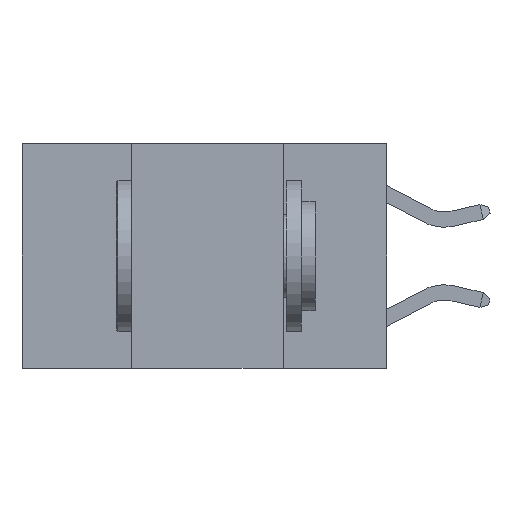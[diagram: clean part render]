
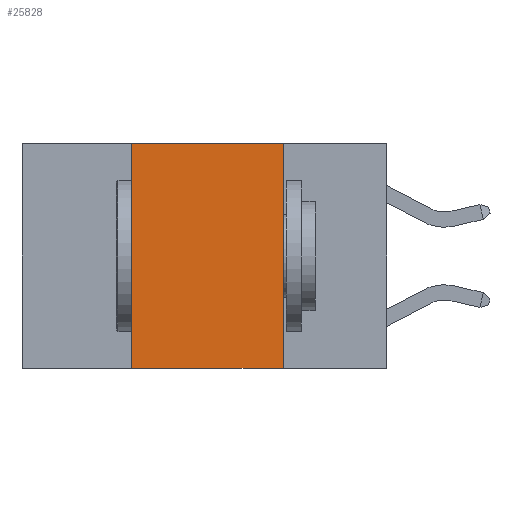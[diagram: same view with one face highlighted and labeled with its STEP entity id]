
A CAD part, left-side view. The second image highlights one B-rep face of the part: STEP entity #25828.
In plain terms, the highlighted planar face has unit normal (-1, 0, 0).
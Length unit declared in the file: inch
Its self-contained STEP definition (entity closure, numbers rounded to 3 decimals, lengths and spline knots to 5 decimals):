
#1135 = ORIENTED_EDGE ( 'NONE', *, *, #9739, .F. ) ;
#1150 = VERTEX_POINT ( 'NONE', #23012 ) ;
#1976 = DIRECTION ( 'NONE',  ( 0., 0., -1. ) ) ;
#2489 = CARTESIAN_POINT ( 'NONE',  ( 0., 0.42, 0. ) ) ;
#2857 = CARTESIAN_POINT ( 'NONE',  ( 0., 0.17, 0. ) ) ;
#2984 = CARTESIAN_POINT ( 'NONE',  ( 0., 0.17, -0.37 ) ) ;
#3422 = VECTOR ( 'NONE', #10357, 39.37008 ) ;
#3441 = ORIENTED_EDGE ( 'NONE', *, *, #26865, .T. ) ;
#4507 = CARTESIAN_POINT ( 'NONE',  ( 0., 0.6, 0. ) ) ;
#5641 = VECTOR ( 'NONE', #6205, 39.37008 ) ;
#6205 = DIRECTION ( 'NONE',  ( 0., -1., 0. ) ) ;
#6783 = CARTESIAN_POINT ( 'NONE',  ( 0., 0.6, 0. ) ) ;
#6933 = DIRECTION ( 'NONE',  ( 0., -1., 0. ) ) ;
#7916 = CARTESIAN_POINT ( 'NONE',  ( 0., 0.17, 0. ) ) ;
#8054 = EDGE_LOOP ( 'NONE', ( #18861, #1135, #26654, #3441 ) ) ;
#9739 = EDGE_CURVE ( 'NONE', #22790, #9979, #10816, .T. ) ;
#9979 = VERTEX_POINT ( 'NONE', #2857 ) ;
#10357 = DIRECTION ( 'NONE',  ( 0., 0., -1. ) ) ;
#10816 = LINE ( 'NONE', #4507, #27538 ) ;
#14613 = VERTEX_POINT ( 'NONE', #2984 ) ;
#16441 = DIRECTION ( 'NONE',  ( 1., 0., 0. ) ) ;
#16897 = LINE ( 'NONE', #20516, #5641 ) ;
#16934 = AXIS2_PLACEMENT_3D ( 'NONE', #6783, #16441, #1976 ) ;
#18861 = ORIENTED_EDGE ( 'NONE', *, *, #21683, .F. ) ;
#19309 = DIRECTION ( 'NONE',  ( 0., 0., 1. ) ) ;
#20516 = CARTESIAN_POINT ( 'NONE',  ( 0., 0.6, -0.37 ) ) ;
#21041 = FACE_OUTER_BOUND ( 'NONE', #8054, .T. ) ;
#21683 = EDGE_CURVE ( 'NONE', #9979, #14613, #22578, .T. ) ;
#22578 = LINE ( 'NONE', #7916, #3422 ) ;
#22790 = VERTEX_POINT ( 'NONE', #23615 ) ;
#23012 = CARTESIAN_POINT ( 'NONE',  ( 0., 0.42, -0.37 ) ) ;
#23474 = EDGE_CURVE ( 'NONE', #1150, #22790, #29096, .T. ) ;
#23565 = VECTOR ( 'NONE', #19309, 39.37008 ) ;
#23615 = CARTESIAN_POINT ( 'NONE',  ( 0., 0.42, 0. ) ) ;
#25828 = ADVANCED_FACE ( 'NONE', ( #21041 ), #28234, .F. ) ;
#26654 = ORIENTED_EDGE ( 'NONE', *, *, #23474, .F. ) ;
#26865 = EDGE_CURVE ( 'NONE', #1150, #14613, #16897, .T. ) ;
#27538 = VECTOR ( 'NONE', #6933, 39.37008 ) ;
#28234 = PLANE ( 'NONE',  #16934 ) ;
#29096 = LINE ( 'NONE', #2489, #23565 ) ;
